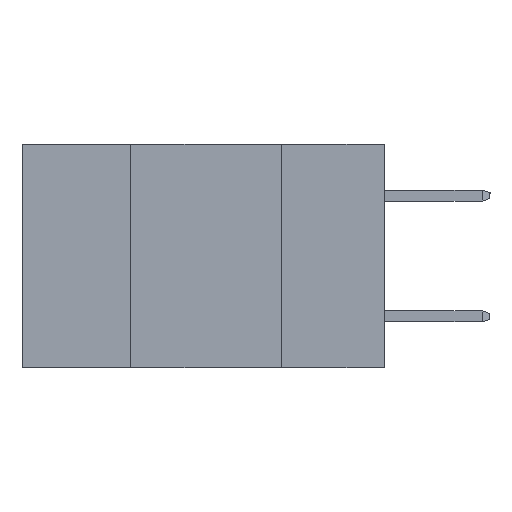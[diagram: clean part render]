
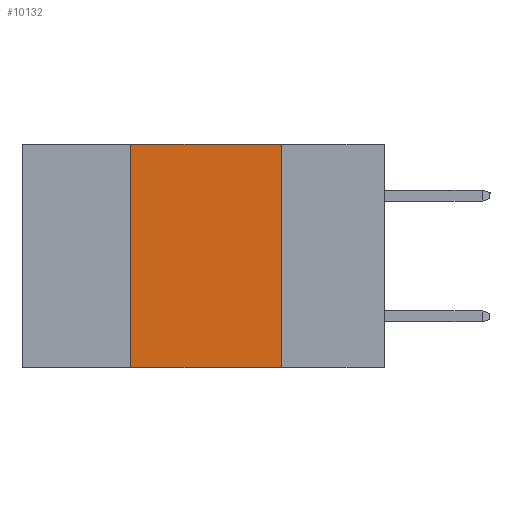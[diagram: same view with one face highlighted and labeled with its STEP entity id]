
A CAD part, left-side view. The second image highlights one B-rep face of the part: STEP entity #10132.
In plain terms, the highlighted planar face has unit normal (-1, 0, 0).
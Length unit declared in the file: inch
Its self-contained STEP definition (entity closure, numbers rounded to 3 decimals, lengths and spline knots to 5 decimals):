
#117 = VERTEX_POINT ( 'NONE', #9372 ) ;
#139 = VERTEX_POINT ( 'NONE', #1753 ) ;
#550 = CARTESIAN_POINT ( 'NONE',  ( 0., 0.17, 0. ) ) ;
#621 = ORIENTED_EDGE ( 'NONE', *, *, #15597, .F. ) ;
#1086 = CARTESIAN_POINT ( 'NONE',  ( 0., 0.6, -0.37 ) ) ;
#1119 = CARTESIAN_POINT ( 'NONE',  ( 0., 0.6, 0. ) ) ;
#1753 = CARTESIAN_POINT ( 'NONE',  ( 0., 0.17, -0.37 ) ) ;
#1877 = LINE ( 'NONE', #3368, #14040 ) ;
#2494 = VECTOR ( 'NONE', #6224, 39.37008 ) ;
#2581 = CARTESIAN_POINT ( 'NONE',  ( 0., 0.17, -0.37 ) ) ;
#2696 = EDGE_CURVE ( 'NONE', #117, #139, #12571, .T. ) ;
#3368 = CARTESIAN_POINT ( 'NONE',  ( 0., 0.6, 0. ) ) ;
#3878 = ORIENTED_EDGE ( 'NONE', *, *, #15095, .F. ) ;
#4819 = EDGE_CURVE ( 'NONE', #7107, #13547, #1877, .T. ) ;
#4968 = DIRECTION ( 'NONE',  ( 1., 0., 0. ) ) ;
#5145 = DIRECTION ( 'NONE',  ( 0., 0., -1. ) ) ;
#5786 = VECTOR ( 'NONE', #5145, 39.37008 ) ;
#6069 = FACE_OUTER_BOUND ( 'NONE', #9961, .T. ) ;
#6170 = PLANE ( 'NONE',  #14299 ) ;
#6224 = DIRECTION ( 'NONE',  ( 0., -1., 0. ) ) ;
#7107 = VERTEX_POINT ( 'NONE', #9203 ) ;
#7977 = DIRECTION ( 'NONE',  ( 0., 0., 1. ) ) ;
#9203 = CARTESIAN_POINT ( 'NONE',  ( 0., 0.42, 0. ) ) ;
#9238 = CARTESIAN_POINT ( 'NONE',  ( 0., 0.42, -0.37 ) ) ;
#9372 = CARTESIAN_POINT ( 'NONE',  ( 0., 0.42, -0.37 ) ) ;
#9961 = EDGE_LOOP ( 'NONE', ( #3878, #13651, #621, #16352 ) ) ;
#10090 = DIRECTION ( 'NONE',  ( 0., 0., -1. ) ) ;
#10119 = LINE ( 'NONE', #2581, #5786 ) ;
#10132 = ADVANCED_FACE ( 'NONE', ( #6069 ), #6170, .F. ) ;
#11961 = VECTOR ( 'NONE', #7977, 39.37008 ) ;
#12571 = LINE ( 'NONE', #1086, #2494 ) ;
#13547 = VERTEX_POINT ( 'NONE', #550 ) ;
#13651 = ORIENTED_EDGE ( 'NONE', *, *, #4819, .F. ) ;
#14040 = VECTOR ( 'NONE', #14795, 39.37008 ) ;
#14286 = LINE ( 'NONE', #9238, #11961 ) ;
#14299 = AXIS2_PLACEMENT_3D ( 'NONE', #1119, #4968, #10090 ) ;
#14795 = DIRECTION ( 'NONE',  ( 0., -1., 0. ) ) ;
#15095 = EDGE_CURVE ( 'NONE', #13547, #139, #10119, .T. ) ;
#15597 = EDGE_CURVE ( 'NONE', #117, #7107, #14286, .T. ) ;
#16352 = ORIENTED_EDGE ( 'NONE', *, *, #2696, .T. ) ;
